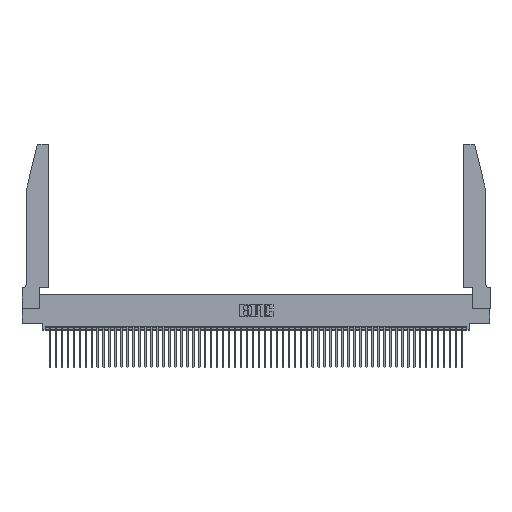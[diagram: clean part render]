
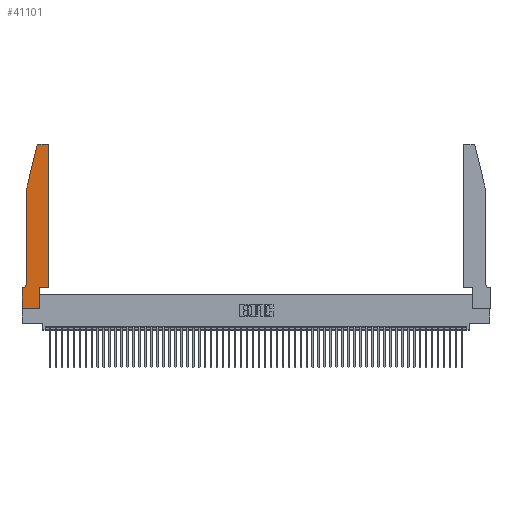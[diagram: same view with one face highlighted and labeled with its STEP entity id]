
A CAD part, top view. The second image highlights one B-rep face of the part: STEP entity #41101.
In plain terms, the highlighted planar face has unit normal (0, 0, 1).
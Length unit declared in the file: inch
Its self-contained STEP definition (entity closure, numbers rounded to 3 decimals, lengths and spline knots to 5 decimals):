
#511 = LINE ( 'NONE', #20624, #33910 ) ;
#679 = CARTESIAN_POINT ( 'NONE',  ( 0.4505, 0.35, 0.37 ) ) ;
#1545 = CARTESIAN_POINT ( 'NONE',  ( 0.2865, 0., 0.37 ) ) ;
#2606 = LINE ( 'NONE', #5106, #46006 ) ;
#2725 = EDGE_CURVE ( 'NONE', #47178, #30414, #21164, .T. ) ;
#2925 = LINE ( 'NONE', #5151, #46327 ) ;
#3632 = CARTESIAN_POINT ( 'NONE',  ( 0., 0., 0.37 ) ) ;
#3788 = ORIENTED_EDGE ( 'NONE', *, *, #34197, .T. ) ;
#5106 = CARTESIAN_POINT ( 'NONE',  ( 0.4505, 0.35, 0.37 ) ) ;
#5151 = CARTESIAN_POINT ( 'NONE',  ( 0., 0., 0.37 ) ) ;
#5380 = CARTESIAN_POINT ( 'NONE',  ( 0.2865, 0.35, 0.37 ) ) ;
#6143 = ORIENTED_EDGE ( 'NONE', *, *, #14181, .T. ) ;
#6305 = CARTESIAN_POINT ( 'NONE',  ( 0., 0., 0.37 ) ) ;
#6874 = EDGE_CURVE ( 'NONE', #43757, #45624, #44405, .T. ) ;
#7558 = DIRECTION ( 'NONE',  ( 0., -1., 0. ) ) ;
#8795 = FACE_OUTER_BOUND ( 'NONE', #14186, .T. ) ;
#9222 = VERTEX_POINT ( 'NONE', #6305 ) ;
#9536 = DIRECTION ( 'NONE',  ( -0.239, -0.971, 0. ) ) ;
#9595 = DIRECTION ( 'NONE',  ( 0., 1., 0. ) ) ;
#9851 = DIRECTION ( 'NONE',  ( -1., 0., 0. ) ) ;
#10231 = CARTESIAN_POINT ( 'NONE',  ( 0.284, 2.75, 0.37 ) ) ;
#11201 = VERTEX_POINT ( 'NONE', #19639 ) ;
#12509 = DIRECTION ( 'NONE',  ( 0., -1., 0. ) ) ;
#12646 = LINE ( 'NONE', #39543, #34273 ) ;
#13590 = VERTEX_POINT ( 'NONE', #10231 ) ;
#13973 = DIRECTION ( 'NONE',  ( 1., 0., 0. ) ) ;
#14181 = EDGE_CURVE ( 'NONE', #21035, #50468, #2606, .T. ) ;
#14186 = EDGE_LOOP ( 'NONE', ( #38622, #40363, #27850, #44404, #3788, #27153, #34780, #42477, #28875, #23961, #6143, #34021 ) ) ;
#14536 = CARTESIAN_POINT ( 'NONE',  ( 0.4205, 2.72, 0.37 ) ) ;
#16051 = DIRECTION ( 'NONE',  ( 0., 0., 1. ) ) ;
#17788 = CARTESIAN_POINT ( 'NONE',  ( 0.2865, 0.35, 0.37 ) ) ;
#18424 = CARTESIAN_POINT ( 'NONE',  ( 0.4505, 2.72, 0.37 ) ) ;
#18541 = CARTESIAN_POINT ( 'NONE',  ( 0.0755, 0.35, 0.37 ) ) ;
#18872 = DIRECTION ( 'NONE',  ( 1., 0., 0. ) ) ;
#19011 = DIRECTION ( 'NONE',  ( 0., 0., -1. ) ) ;
#19639 = CARTESIAN_POINT ( 'NONE',  ( 0.0055, 0.35, 0.37 ) ) ;
#20239 = EDGE_CURVE ( 'NONE', #23096, #9222, #50789, .T. ) ;
#20624 = CARTESIAN_POINT ( 'NONE',  ( 0.2605, 2.75, 0.37 ) ) ;
#21035 = VERTEX_POINT ( 'NONE', #52775 ) ;
#21164 = LINE ( 'NONE', #42168, #31329 ) ;
#22486 = EDGE_CURVE ( 'NONE', #11201, #23096, #36982, .T. ) ;
#22785 = AXIS2_PLACEMENT_3D ( 'NONE', #14536, #44701, #18872 ) ;
#23096 = VERTEX_POINT ( 'NONE', #31725 ) ;
#23336 = DIRECTION ( 'NONE',  ( 0., 0., 1. ) ) ;
#23961 = ORIENTED_EDGE ( 'NONE', *, *, #52184, .T. ) ;
#26646 = CIRCLE ( 'NONE', #22785, 0.03 ) ;
#26899 = CIRCLE ( 'NONE', #30056, 0.07 ) ;
#27028 = CIRCLE ( 'NONE', #46908, 0.03 ) ;
#27153 = ORIENTED_EDGE ( 'NONE', *, *, #22486, .T. ) ;
#27771 = CARTESIAN_POINT ( 'NONE',  ( 0.0755, 0.42, 0.37 ) ) ;
#27850 = ORIENTED_EDGE ( 'NONE', *, *, #31629, .T. ) ;
#28875 = ORIENTED_EDGE ( 'NONE', *, *, #6874, .T. ) ;
#29699 = EDGE_CURVE ( 'NONE', #13590, #35736, #27028, .T. ) ;
#30056 = AXIS2_PLACEMENT_3D ( 'NONE', #44845, #19011, #49177 ) ;
#30414 = VERTEX_POINT ( 'NONE', #27771 ) ;
#31329 = VECTOR ( 'NONE', #7558, 39.37008 ) ;
#31621 = VECTOR ( 'NONE', #34781, 39.37008 ) ;
#31629 = EDGE_CURVE ( 'NONE', #35736, #47178, #12646, .T. ) ;
#31725 = CARTESIAN_POINT ( 'NONE',  ( 0., 0.35, 0.37 ) ) ;
#32863 = EDGE_CURVE ( 'NONE', #50468, #55365, #26646, .T. ) ;
#33910 = VECTOR ( 'NONE', #50795, 39.37008 ) ;
#34021 = ORIENTED_EDGE ( 'NONE', *, *, #32863, .T. ) ;
#34197 = EDGE_CURVE ( 'NONE', #30414, #11201, #26899, .T. ) ;
#34273 = VECTOR ( 'NONE', #9536, 39.37008 ) ;
#34780 = ORIENTED_EDGE ( 'NONE', *, *, #20239, .T. ) ;
#34781 = DIRECTION ( 'NONE',  ( 0., 1., 0. ) ) ;
#35349 = VECTOR ( 'NONE', #13973, 39.37008 ) ;
#35736 = VERTEX_POINT ( 'NONE', #50740 ) ;
#36164 = CARTESIAN_POINT ( 'NONE',  ( 0., 0.35, 0.37 ) ) ;
#36982 = LINE ( 'NONE', #18541, #47077 ) ;
#38622 = ORIENTED_EDGE ( 'NONE', *, *, #45404, .T. ) ;
#38672 = EDGE_CURVE ( 'NONE', #9222, #43757, #2925, .T. ) ;
#39324 = VECTOR ( 'NONE', #12509, 39.37008 ) ;
#39543 = CARTESIAN_POINT ( 'NONE',  ( 0.0755, 2., 0.37 ) ) ;
#40363 = ORIENTED_EDGE ( 'NONE', *, *, #29699, .T. ) ;
#41101 = ADVANCED_FACE ( 'NONE', ( #8795 ), #49148, .T. ) ;
#41452 = AXIS2_PLACEMENT_3D ( 'NONE', #36164, #23336, #53484 ) ;
#41870 = CARTESIAN_POINT ( 'NONE',  ( 0.284, 2.72, 0.37 ) ) ;
#41966 = CARTESIAN_POINT ( 'NONE',  ( 0.0755, 2., 0.37 ) ) ;
#42168 = CARTESIAN_POINT ( 'NONE',  ( 0.0755, 2., 0.37 ) ) ;
#42477 = ORIENTED_EDGE ( 'NONE', *, *, #38672, .T. ) ;
#43757 = VERTEX_POINT ( 'NONE', #1545 ) ;
#43976 = DIRECTION ( 'NONE',  ( 1., 0., 0. ) ) ;
#44404 = ORIENTED_EDGE ( 'NONE', *, *, #2725, .T. ) ;
#44405 = LINE ( 'NONE', #17788, #31621 ) ;
#44701 = DIRECTION ( 'NONE',  ( 0., 0., 1. ) ) ;
#44845 = CARTESIAN_POINT ( 'NONE',  ( 0.0055, 0.42, 0.37 ) ) ;
#45404 = EDGE_CURVE ( 'NONE', #55365, #13590, #511, .T. ) ;
#45624 = VERTEX_POINT ( 'NONE', #5380 ) ;
#46006 = VECTOR ( 'NONE', #9595, 39.37008 ) ;
#46188 = DIRECTION ( 'NONE',  ( 1., 0., 0. ) ) ;
#46327 = VECTOR ( 'NONE', #43976, 39.37008 ) ;
#46804 = LINE ( 'NONE', #679, #35349 ) ;
#46908 = AXIS2_PLACEMENT_3D ( 'NONE', #41870, #16051, #46188 ) ;
#47077 = VECTOR ( 'NONE', #9851, 39.37008 ) ;
#47178 = VERTEX_POINT ( 'NONE', #41966 ) ;
#49148 = PLANE ( 'NONE',  #41452 ) ;
#49177 = DIRECTION ( 'NONE',  ( -1., 0., 0. ) ) ;
#50468 = VERTEX_POINT ( 'NONE', #18424 ) ;
#50740 = CARTESIAN_POINT ( 'NONE',  ( 0.25487, 2.72718, 0.37 ) ) ;
#50789 = LINE ( 'NONE', #3632, #39324 ) ;
#50795 = DIRECTION ( 'NONE',  ( -1., 0., 0. ) ) ;
#52184 = EDGE_CURVE ( 'NONE', #45624, #21035, #46804, .T. ) ;
#52775 = CARTESIAN_POINT ( 'NONE',  ( 0.4505, 0.35, 0.37 ) ) ;
#53484 = DIRECTION ( 'NONE',  ( 1., 0., 0. ) ) ;
#55365 = VERTEX_POINT ( 'NONE', #55507 ) ;
#55507 = CARTESIAN_POINT ( 'NONE',  ( 0.4205, 2.75, 0.37 ) ) ;
